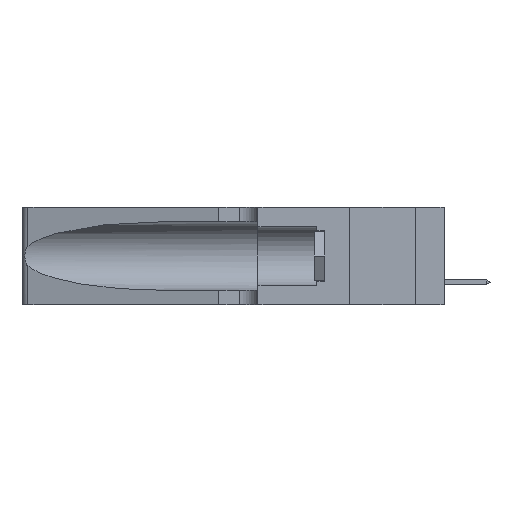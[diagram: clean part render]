
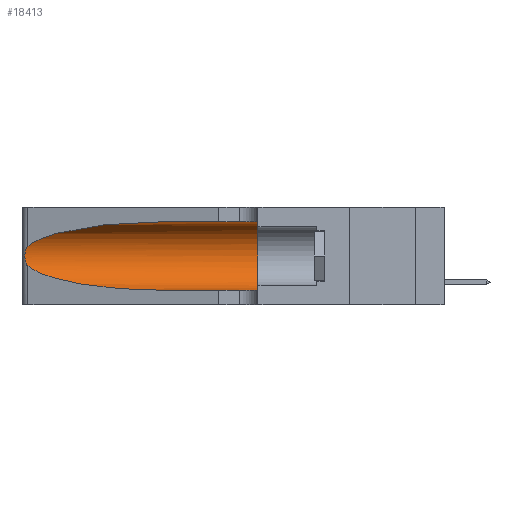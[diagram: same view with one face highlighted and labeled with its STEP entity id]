
A CAD part, left-side view. The second image highlights one B-rep face of the part: STEP entity #18413.
In plain terms, the highlighted cylindrical face has radius 3.308 mm (diameter 6.617 mm), a partial arc.
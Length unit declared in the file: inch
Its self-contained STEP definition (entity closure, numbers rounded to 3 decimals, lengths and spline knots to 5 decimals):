
#481 = EDGE_LOOP ( 'NONE', ( #29997, #5798, #17884, #5923, #31678, #14728 ) ) ;
#941 = EDGE_CURVE ( 'NONE', #19357, #5463, #26582, .T. ) ;
#2803 = CARTESIAN_POINT ( 'NONE',  ( 0.1305, 0.72297, 0.05475 ) ) ;
#2984 = CARTESIAN_POINT ( 'NONE',  ( 0.18966, 0.96281, 0.31525 ) ) ;
#3653 = DIRECTION ( 'NONE',  ( 0., 0., -1. ) ) ;
#4114 = VECTOR ( 'NONE', #25978, 39.37008 ) ;
#5463 = VERTEX_POINT ( 'NONE', #22412 ) ;
#5699 = CARTESIAN_POINT ( 'NONE',  ( 0.25487, 1.22718, 0.22369 ) ) ;
#5798 = ORIENTED_EDGE ( 'NONE', *, *, #9902, .T. ) ;
#5923 = ORIENTED_EDGE ( 'NONE', *, *, #941, .T. ) ;
#6089 = CARTESIAN_POINT ( 'NONE',  ( 0.25487, 1.22718, 0.22369 ) ) ;
#6202 = CARTESIAN_POINT ( 'NONE',  ( 0.25639, 1.23186, 0.15144 ) ) ;
#6575 = CARTESIAN_POINT ( 'NONE',  ( 0.1305, 1.61858, 0.05475 ) ) ;
#8041 = VERTEX_POINT ( 'NONE', #18106 ) ;
#8475 = CARTESIAN_POINT ( 'NONE',  ( 0.26018, 1.23835, 0.19895 ) ) ;
#8807 = CARTESIAN_POINT ( 'NONE',  ( 0.25555, 1.22993, 0.14849 ) ) ;
#9902 = EDGE_CURVE ( 'NONE', #13867, #8041, #30139, .T. ) ;
#10652 = LINE ( 'NONE', #28875, #11071 ) ;
#11026 = CARTESIAN_POINT ( 'NONE',  ( 0.1305, 1.61858, 0.185 ) ) ;
#11071 = VECTOR ( 'NONE', #11528, 39.37008 ) ;
#11528 = DIRECTION ( 'NONE',  ( 0., -1., 0. ) ) ;
#11783 = CIRCLE ( 'NONE', #22799, 0.13025 ) ;
#12342 = AXIS2_PLACEMENT_3D ( 'NONE', #11026, #28359, #3653 ) ;
#12764 = FACE_OUTER_BOUND ( 'NONE', #481, .T. ) ;
#13811 = CARTESIAN_POINT ( 'NONE',  ( 0.25854, 1.2359, 0.20912 ) ) ;
#13867 = VERTEX_POINT ( 'NONE', #15595 ) ;
#13911 = CARTESIAN_POINT ( 'NONE',  ( 0.26017, 1.23833, 0.17102 ) ) ;
#14281 =( BOUNDED_CURVE ( )  B_SPLINE_CURVE ( 3, ( #17742, #2984, #20397, #5699 ),
 .UNSPECIFIED., .F., .T. ) 
 B_SPLINE_CURVE_WITH_KNOTS ( ( 4, 4 ),
 ( 1.5708, 2.84003 ),
 .UNSPECIFIED. ) 
 CURVE ( )  GEOMETRIC_REPRESENTATION_ITEM ( )  RATIONAL_B_SPLINE_CURVE ( ( 1., 0.87, 0.87, 1. ) ) 
 REPRESENTATION_ITEM ( '' )  );
#14657 = CARTESIAN_POINT ( 'NONE',  ( 0.2373, 1.15595, 0.08982 ) ) ;
#14728 = ORIENTED_EDGE ( 'NONE', *, *, #24284, .F. ) ;
#14862 = VERTEX_POINT ( 'NONE', #21050 ) ;
#15144 = DIRECTION ( 'NONE',  ( 0., 0., 1. ) ) ;
#15595 = CARTESIAN_POINT ( 'NONE',  ( 0.25487, 1.22718, 0.22369 ) ) ;
#15646 = EDGE_CURVE ( 'NONE', #22196, #5463, #11783, .T. ) ;
#15949 = CARTESIAN_POINT ( 'NONE',  ( 0.26075, 1.23896, 0.178 ) ) ;
#16267 = CYLINDRICAL_SURFACE ( 'NONE', #12342, 0.13025 ) ;
#16404 = CARTESIAN_POINT ( 'NONE',  ( 0.25555, 1.22994, 0.2215 ) ) ;
#17742 = CARTESIAN_POINT ( 'NONE',  ( 0.1305, 0.72297, 0.31525 ) ) ;
#17884 = ORIENTED_EDGE ( 'NONE', *, *, #19181, .T. ) ;
#18106 = CARTESIAN_POINT ( 'NONE',  ( 0.25487, 1.22718, 0.14631 ) ) ;
#18413 = ADVANCED_FACE ( 'NONE', ( #12764 ), #16267, .F. ) ;
#18653 =( BOUNDED_CURVE ( )  B_SPLINE_CURVE ( 3, ( #27005, #14657, #32027, #2803 ),
 .UNSPECIFIED., .F., .F. ) 
 B_SPLINE_CURVE_WITH_KNOTS ( ( 4, 4 ),
 ( 3.44316, 4.71239 ),
 .UNSPECIFIED. ) 
 CURVE ( )  GEOMETRIC_REPRESENTATION_ITEM ( )  RATIONAL_B_SPLINE_CURVE ( ( 1., 0.87, 0.87, 1. ) ) 
 REPRESENTATION_ITEM ( '' )  );
#18660 = EDGE_CURVE ( 'NONE', #14862, #13867, #14281, .T. ) ;
#18688 = CARTESIAN_POINT ( 'NONE',  ( 0.25639, 1.23184, 0.21858 ) ) ;
#19181 = EDGE_CURVE ( 'NONE', #8041, #19357, #18653, .T. ) ;
#19357 = VERTEX_POINT ( 'NONE', #28037 ) ;
#20397 = CARTESIAN_POINT ( 'NONE',  ( 0.2373, 1.15595, 0.28018 ) ) ;
#21050 = CARTESIAN_POINT ( 'NONE',  ( 0.1305, 0.72297, 0.31525 ) ) ;
#22196 = VERTEX_POINT ( 'NONE', #25316 ) ;
#22412 = CARTESIAN_POINT ( 'NONE',  ( 0.1305, 0.35, 0.05475 ) ) ;
#22799 = AXIS2_PLACEMENT_3D ( 'NONE', #23038, #25123, #15144 ) ;
#23038 = CARTESIAN_POINT ( 'NONE',  ( 0.1305, 0.35, 0.185 ) ) ;
#23281 = CARTESIAN_POINT ( 'NONE',  ( 0.25787, 1.23484, 0.2124 ) ) ;
#24284 = EDGE_CURVE ( 'NONE', #14862, #22196, #10652, .T. ) ;
#25123 = DIRECTION ( 'NONE',  ( 0., 1., 0. ) ) ;
#25316 = CARTESIAN_POINT ( 'NONE',  ( 0.1305, 0.35, 0.31525 ) ) ;
#25814 = CARTESIAN_POINT ( 'NONE',  ( 0.25856, 1.23593, 0.16098 ) ) ;
#25978 = DIRECTION ( 'NONE',  ( 0., -1., 0. ) ) ;
#26036 = CARTESIAN_POINT ( 'NONE',  ( 0.26075, 1.23896, 0.19203 ) ) ;
#26582 = LINE ( 'NONE', #6575, #4114 ) ;
#27005 = CARTESIAN_POINT ( 'NONE',  ( 0.25487, 1.22718, 0.14631 ) ) ;
#28037 = CARTESIAN_POINT ( 'NONE',  ( 0.1305, 0.72297, 0.05475 ) ) ;
#28359 = DIRECTION ( 'NONE',  ( 0., -1., 0. ) ) ;
#28418 = CARTESIAN_POINT ( 'NONE',  ( 0.25789, 1.23486, 0.15765 ) ) ;
#28875 = CARTESIAN_POINT ( 'NONE',  ( 0.1305, 1.61858, 0.31525 ) ) ;
#29997 = ORIENTED_EDGE ( 'NONE', *, *, #18660, .T. ) ;
#30139 = B_SPLINE_CURVE_WITH_KNOTS ( 'NONE', 3,
 ( #6089, #16404, #18688, #23281, #13811, #8475, #26036, #15949, #13911, #25814, #28418, #6202, #8807, #31149 ),
 .UNSPECIFIED., .F., .F.,
 ( 4, 2, 2, 2, 2, 2, 4 ),
 ( 0., 0.00027, 0.00053, 0.00107, 0.0016, 0.00187, 0.00214 ),
 .UNSPECIFIED. ) ;
#31149 = CARTESIAN_POINT ( 'NONE',  ( 0.25487, 1.22718, 0.14631 ) ) ;
#31678 = ORIENTED_EDGE ( 'NONE', *, *, #15646, .F. ) ;
#32027 = CARTESIAN_POINT ( 'NONE',  ( 0.18966, 0.96281, 0.05475 ) ) ;
